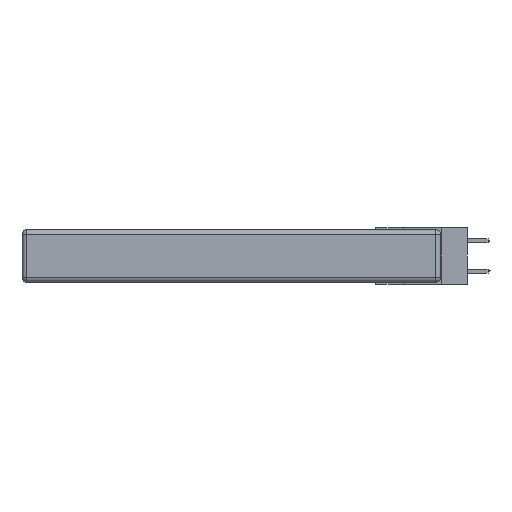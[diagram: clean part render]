
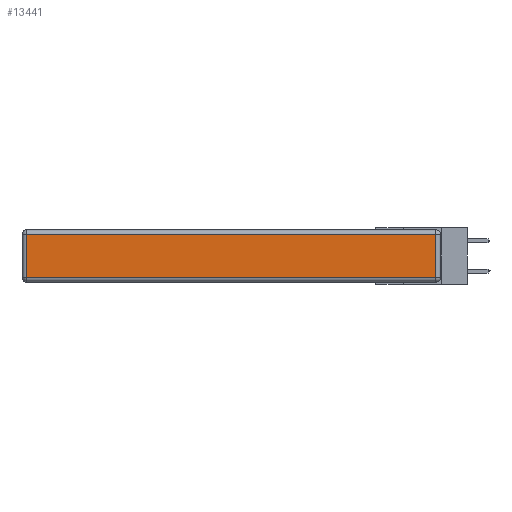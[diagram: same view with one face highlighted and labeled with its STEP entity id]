
A CAD part, left-side view. The second image highlights one B-rep face of the part: STEP entity #13441.
In plain terms, the highlighted planar face has unit normal (-1, 0, 0).
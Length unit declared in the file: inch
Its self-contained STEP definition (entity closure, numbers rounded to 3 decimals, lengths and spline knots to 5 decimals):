
#582 = VERTEX_POINT ( 'NONE', #6305 ) ;
#1106 = CARTESIAN_POINT ( 'NONE',  ( 0., 2.72, -0.343 ) ) ;
#1481 = CARTESIAN_POINT ( 'NONE',  ( 0., 0.03, -0.343 ) ) ;
#1549 = VERTEX_POINT ( 'NONE', #6392 ) ;
#1587 = LINE ( 'NONE', #9055, #7268 ) ;
#2261 = VERTEX_POINT ( 'NONE', #5526 ) ;
#2353 = EDGE_CURVE ( 'NONE', #2261, #1549, #10324, .T. ) ;
#2543 = LINE ( 'NONE', #6558, #12217 ) ;
#3127 = DIRECTION ( 'NONE',  ( 0., 1., 0. ) ) ;
#4195 = PLANE ( 'NONE',  #9878 ) ;
#4237 = DIRECTION ( 'NONE',  ( 0., 0., 1. ) ) ;
#4759 = EDGE_LOOP ( 'NONE', ( #14000, #7253, #9889, #7591 ) ) ;
#4883 = EDGE_CURVE ( 'NONE', #13952, #2261, #2543, .T. ) ;
#5339 = DIRECTION ( 'NONE',  ( -1., 0., 0. ) ) ;
#5526 = CARTESIAN_POINT ( 'NONE',  ( 0., 0.03, -0.313 ) ) ;
#6305 = CARTESIAN_POINT ( 'NONE',  ( 0., 2.72, -0.03 ) ) ;
#6392 = CARTESIAN_POINT ( 'NONE',  ( 0., 0.03, -0.03 ) ) ;
#6558 = CARTESIAN_POINT ( 'NONE',  ( 0., 0., -0.313 ) ) ;
#6915 = EDGE_CURVE ( 'NONE', #1549, #582, #1587, .T. ) ;
#7253 = ORIENTED_EDGE ( 'NONE', *, *, #2353, .T. ) ;
#7268 = VECTOR ( 'NONE', #3127, 39.37008 ) ;
#7591 = ORIENTED_EDGE ( 'NONE', *, *, #8709, .T. ) ;
#7932 = LINE ( 'NONE', #1106, #12640 ) ;
#8709 = EDGE_CURVE ( 'NONE', #582, #13952, #7932, .T. ) ;
#9055 = CARTESIAN_POINT ( 'NONE',  ( 0., 2.75, -0.03 ) ) ;
#9878 = AXIS2_PLACEMENT_3D ( 'NONE', #14646, #5339, #4237 ) ;
#9889 = ORIENTED_EDGE ( 'NONE', *, *, #6915, .T. ) ;
#10324 = LINE ( 'NONE', #1481, #14477 ) ;
#12217 = VECTOR ( 'NONE', #14614, 39.37008 ) ;
#12381 = CARTESIAN_POINT ( 'NONE',  ( 0., 2.72, -0.313 ) ) ;
#12513 = DIRECTION ( 'NONE',  ( 0., 0., -1. ) ) ;
#12640 = VECTOR ( 'NONE', #12513, 39.37008 ) ;
#12801 = DIRECTION ( 'NONE',  ( 0., 0., 1. ) ) ;
#13441 = ADVANCED_FACE ( 'NONE', ( #13676 ), #4195, .T. ) ;
#13676 = FACE_OUTER_BOUND ( 'NONE', #4759, .T. ) ;
#13952 = VERTEX_POINT ( 'NONE', #12381 ) ;
#14000 = ORIENTED_EDGE ( 'NONE', *, *, #4883, .T. ) ;
#14477 = VECTOR ( 'NONE', #12801, 39.37008 ) ;
#14614 = DIRECTION ( 'NONE',  ( 0., -1., 0. ) ) ;
#14646 = CARTESIAN_POINT ( 'NONE',  ( 0., 0., -0.343 ) ) ;
